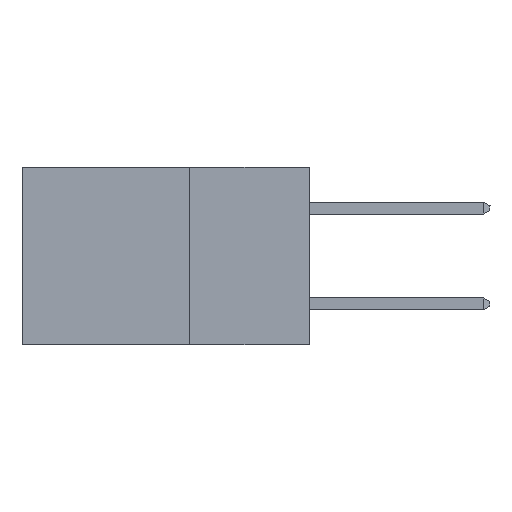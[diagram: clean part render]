
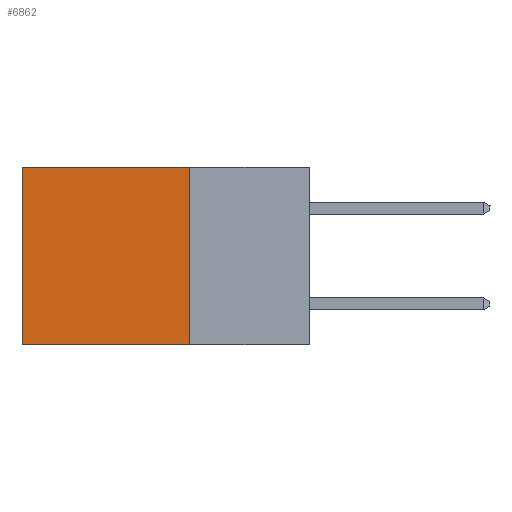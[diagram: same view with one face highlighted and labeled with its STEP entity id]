
A CAD part, left-side view. The second image highlights one B-rep face of the part: STEP entity #6862.
In plain terms, the highlighted planar face has unit normal (-1, 0, 0).
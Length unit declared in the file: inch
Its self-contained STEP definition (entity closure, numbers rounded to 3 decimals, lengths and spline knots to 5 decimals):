
#658 = CARTESIAN_POINT ( 'NONE',  ( 0.2875, 0.25, 0. ) ) ;
#784 = VECTOR ( 'NONE', #10039, 39.37008 ) ;
#849 = LINE ( 'NONE', #1965, #784 ) ;
#1142 = EDGE_CURVE ( 'NONE', #6517, #13981, #3057, .T. ) ;
#1456 = VERTEX_POINT ( 'NONE', #8108 ) ;
#1571 = CARTESIAN_POINT ( 'NONE',  ( 0.2875, 0.25, -0.37 ) ) ;
#1765 = ORIENTED_EDGE ( 'NONE', *, *, #8480, .T. ) ;
#1810 = CARTESIAN_POINT ( 'NONE',  ( 0.2875, 0.25, 0. ) ) ;
#1965 = CARTESIAN_POINT ( 'NONE',  ( 0.2875, 0.6, 0. ) ) ;
#2845 = DIRECTION ( 'NONE',  ( 0., 1., 0. ) ) ;
#2861 = EDGE_LOOP ( 'NONE', ( #1765, #9016, #6790, #4281 ) ) ;
#3057 = LINE ( 'NONE', #14011, #6763 ) ;
#3866 = DIRECTION ( 'NONE',  ( 0., 1., 0. ) ) ;
#4135 = DIRECTION ( 'NONE',  ( 1., 0., 0. ) ) ;
#4276 = FACE_OUTER_BOUND ( 'NONE', #2861, .T. ) ;
#4281 = ORIENTED_EDGE ( 'NONE', *, *, #12775, .T. ) ;
#5244 = CARTESIAN_POINT ( 'NONE',  ( 0.2875, 0.25, 0. ) ) ;
#5273 = CARTESIAN_POINT ( 'NONE',  ( 0.2875, 0.6, -0.37 ) ) ;
#5437 = PLANE ( 'NONE',  #7798 ) ;
#5851 = LINE ( 'NONE', #1571, #8274 ) ;
#6332 = DIRECTION ( 'NONE',  ( 0., 0., -1. ) ) ;
#6517 = VERTEX_POINT ( 'NONE', #5244 ) ;
#6763 = VECTOR ( 'NONE', #7241, 39.37008 ) ;
#6790 = ORIENTED_EDGE ( 'NONE', *, *, #1142, .F. ) ;
#6862 = ADVANCED_FACE ( 'NONE', ( #4276 ), #5437, .F. ) ;
#7241 = DIRECTION ( 'NONE',  ( 0., 0., -1. ) ) ;
#7552 = EDGE_CURVE ( 'NONE', #13981, #10092, #5851, .T. ) ;
#7798 = AXIS2_PLACEMENT_3D ( 'NONE', #658, #4135, #6332 ) ;
#8108 = CARTESIAN_POINT ( 'NONE',  ( 0.2875, 0.6, 0. ) ) ;
#8274 = VECTOR ( 'NONE', #3866, 39.37008 ) ;
#8480 = EDGE_CURVE ( 'NONE', #1456, #10092, #849, .T. ) ;
#9016 = ORIENTED_EDGE ( 'NONE', *, *, #7552, .F. ) ;
#9052 = CARTESIAN_POINT ( 'NONE',  ( 0.2875, 0.25, -0.37 ) ) ;
#10039 = DIRECTION ( 'NONE',  ( 0., 0., -1. ) ) ;
#10092 = VERTEX_POINT ( 'NONE', #5273 ) ;
#12775 = EDGE_CURVE ( 'NONE', #6517, #1456, #12919, .T. ) ;
#12824 = VECTOR ( 'NONE', #2845, 39.37008 ) ;
#12919 = LINE ( 'NONE', #1810, #12824 ) ;
#13981 = VERTEX_POINT ( 'NONE', #9052 ) ;
#14011 = CARTESIAN_POINT ( 'NONE',  ( 0.2875, 0.25, 0. ) ) ;
